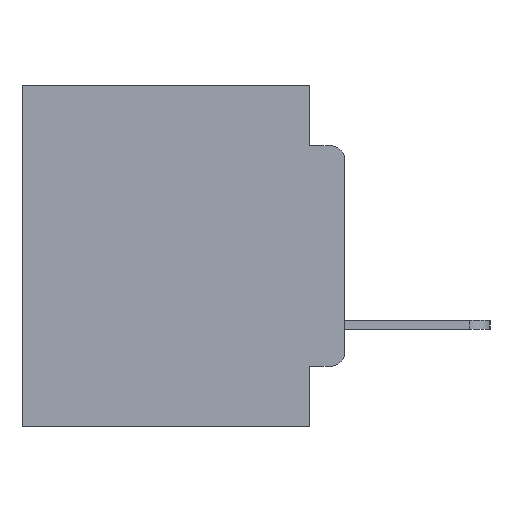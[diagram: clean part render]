
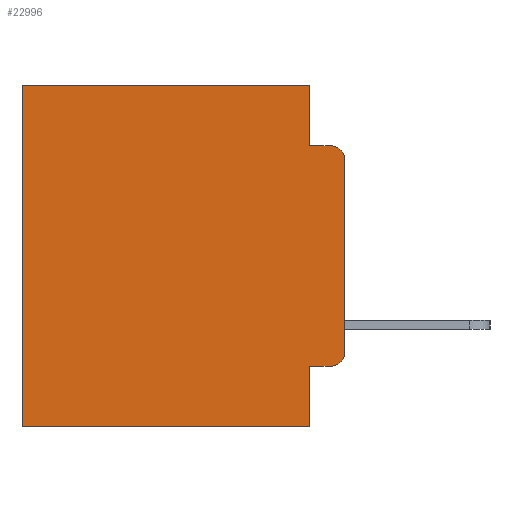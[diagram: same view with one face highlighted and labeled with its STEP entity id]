
A CAD part, left-side view. The second image highlights one B-rep face of the part: STEP entity #22996.
In plain terms, the highlighted planar face has unit normal (-1, 0, 0).
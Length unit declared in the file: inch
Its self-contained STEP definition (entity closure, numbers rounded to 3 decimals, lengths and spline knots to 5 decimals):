
#23 = VERTEX_POINT ( 'NONE', #1239 ) ;
#442 = CARTESIAN_POINT ( 'NONE',  ( 0.298, 0., 0. ) ) ;
#570 = ORIENTED_EDGE ( 'NONE', *, *, #21115, .T. ) ;
#1135 = DIRECTION ( 'NONE',  ( 0., -1., 0. ) ) ;
#1239 = CARTESIAN_POINT ( 'NONE',  ( 0.298, 0.051, -0.5 ) ) ;
#1432 = CARTESIAN_POINT ( 'NONE',  ( 0.298, 0.473, 0. ) ) ;
#1593 = CARTESIAN_POINT ( 'NONE',  ( 0.298, 0., 0. ) ) ;
#1882 = VERTEX_POINT ( 'NONE', #14518 ) ;
#2897 = CARTESIAN_POINT ( 'NONE',  ( 0.298, 0.051, -0.4115 ) ) ;
#2949 = VECTOR ( 'NONE', #7636, 39.37008 ) ;
#3294 = EDGE_CURVE ( 'NONE', #1882, #23, #17187, .T. ) ;
#3575 = VERTEX_POINT ( 'NONE', #11577 ) ;
#3702 = VECTOR ( 'NONE', #11290, 39.37008 ) ;
#5609 = VERTEX_POINT ( 'NONE', #14919 ) ;
#5889 = VERTEX_POINT ( 'NONE', #14248 ) ;
#6291 = CARTESIAN_POINT ( 'NONE',  ( 0.298, 0., -0.5 ) ) ;
#6502 = EDGE_CURVE ( 'NONE', #13504, #9636, #10635, .T. ) ;
#6533 = DIRECTION ( 'NONE',  ( 0., 0., -1. ) ) ;
#6785 = VECTOR ( 'NONE', #25525, 39.37008 ) ;
#6949 = LINE ( 'NONE', #1432, #23338 ) ;
#7346 = EDGE_LOOP ( 'NONE', ( #13256, #25888, #21569, #10869, #22143, #14944, #15572, #26911, #570, #9827 ) ) ;
#7636 = DIRECTION ( 'NONE',  ( 0., 1., 0. ) ) ;
#8042 = VERTEX_POINT ( 'NONE', #13746 ) ;
#9636 = VERTEX_POINT ( 'NONE', #17808 ) ;
#9827 = ORIENTED_EDGE ( 'NONE', *, *, #24387, .T. ) ;
#9970 = LINE ( 'NONE', #2897, #3702 ) ;
#10318 = DIRECTION ( 'NONE',  ( 0., 0., -1. ) ) ;
#10627 = CARTESIAN_POINT ( 'NONE',  ( 0.298, 0., -0.1085 ) ) ;
#10635 = LINE ( 'NONE', #24215, #12045 ) ;
#10776 = DIRECTION ( 'NONE',  ( 0., 0., -1. ) ) ;
#10869 = ORIENTED_EDGE ( 'NONE', *, *, #6502, .F. ) ;
#11014 = CIRCLE ( 'NONE', #19292, 0.02 ) ;
#11290 = DIRECTION ( 'NONE',  ( 0., -1., 0. ) ) ;
#11460 = VECTOR ( 'NONE', #1135, 39.37008 ) ;
#11577 = CARTESIAN_POINT ( 'NONE',  ( 0.298, 0.473, -0.5 ) ) ;
#11649 = VECTOR ( 'NONE', #23100, 39.37008 ) ;
#12045 = VECTOR ( 'NONE', #20986, 39.37008 ) ;
#12156 = LINE ( 'NONE', #15695, #11460 ) ;
#12810 = VECTOR ( 'NONE', #17911, 39.37008 ) ;
#13256 = ORIENTED_EDGE ( 'NONE', *, *, #20235, .F. ) ;
#13476 = LINE ( 'NONE', #442, #12810 ) ;
#13504 = VERTEX_POINT ( 'NONE', #20116 ) ;
#13746 = CARTESIAN_POINT ( 'NONE',  ( 0.298, 0.473, 0. ) ) ;
#14053 = VERTEX_POINT ( 'NONE', #10627 ) ;
#14248 = CARTESIAN_POINT ( 'NONE',  ( 0.298, 0.02, -0.0885 ) ) ;
#14318 = AXIS2_PLACEMENT_3D ( 'NONE', #15518, #20570, #21226 ) ;
#14518 = CARTESIAN_POINT ( 'NONE',  ( 0.298, 0.051, -0.4115 ) ) ;
#14919 = CARTESIAN_POINT ( 'NONE',  ( 0.298, 0., -0.3915 ) ) ;
#14944 = ORIENTED_EDGE ( 'NONE', *, *, #19282, .T. ) ;
#15074 = LINE ( 'NONE', #6291, #2949 ) ;
#15098 = CIRCLE ( 'NONE', #21481, 0.02 ) ;
#15518 = CARTESIAN_POINT ( 'NONE',  ( 0.298, 0., 0. ) ) ;
#15572 = ORIENTED_EDGE ( 'NONE', *, *, #25044, .F. ) ;
#15695 = CARTESIAN_POINT ( 'NONE',  ( 0.298, 0.051, -0.0885 ) ) ;
#17187 = LINE ( 'NONE', #21419, #11649 ) ;
#17793 = CARTESIAN_POINT ( 'NONE',  ( 0.298, 0.02, -0.4115 ) ) ;
#17808 = CARTESIAN_POINT ( 'NONE',  ( 0.298, 0.051, -0.0885 ) ) ;
#17911 = DIRECTION ( 'NONE',  ( 0., 0., -1. ) ) ;
#18573 = VERTEX_POINT ( 'NONE', #17793 ) ;
#18600 = DIRECTION ( 'NONE',  ( -1., 0., 0. ) ) ;
#18780 = CARTESIAN_POINT ( 'NONE',  ( 0.298, 0.02, -0.1085 ) ) ;
#19282 = EDGE_CURVE ( 'NONE', #8042, #3575, #6949, .T. ) ;
#19292 = AXIS2_PLACEMENT_3D ( 'NONE', #18780, #18600, #6533 ) ;
#19779 = EDGE_CURVE ( 'NONE', #9636, #5889, #12156, .T. ) ;
#20055 = PLANE ( 'NONE',  #14318 ) ;
#20061 = CARTESIAN_POINT ( 'NONE',  ( 0.298, 0.02, -0.3915 ) ) ;
#20116 = CARTESIAN_POINT ( 'NONE',  ( 0.298, 0.051, 0. ) ) ;
#20235 = EDGE_CURVE ( 'NONE', #14053, #5609, #13476, .T. ) ;
#20570 = DIRECTION ( 'NONE',  ( 1., 0., 0. ) ) ;
#20986 = DIRECTION ( 'NONE',  ( 0., 0., -1. ) ) ;
#21115 = EDGE_CURVE ( 'NONE', #1882, #18573, #9970, .T. ) ;
#21226 = DIRECTION ( 'NONE',  ( 0., 0., -1. ) ) ;
#21419 = CARTESIAN_POINT ( 'NONE',  ( 0.298, 0.051, 0. ) ) ;
#21481 = AXIS2_PLACEMENT_3D ( 'NONE', #20061, #25992, #10318 ) ;
#21569 = ORIENTED_EDGE ( 'NONE', *, *, #19779, .F. ) ;
#22143 = ORIENTED_EDGE ( 'NONE', *, *, #25555, .T. ) ;
#22996 = ADVANCED_FACE ( 'NONE', ( #26152 ), #20055, .F. ) ;
#23100 = DIRECTION ( 'NONE',  ( 0., 0., -1. ) ) ;
#23338 = VECTOR ( 'NONE', #10776, 39.37008 ) ;
#24215 = CARTESIAN_POINT ( 'NONE',  ( 0.298, 0.051, 0. ) ) ;
#24387 = EDGE_CURVE ( 'NONE', #18573, #5609, #15098, .T. ) ;
#25044 = EDGE_CURVE ( 'NONE', #23, #3575, #15074, .T. ) ;
#25275 = EDGE_CURVE ( 'NONE', #14053, #5889, #11014, .T. ) ;
#25525 = DIRECTION ( 'NONE',  ( 0., 1., 0. ) ) ;
#25555 = EDGE_CURVE ( 'NONE', #13504, #8042, #26755, .T. ) ;
#25888 = ORIENTED_EDGE ( 'NONE', *, *, #25275, .T. ) ;
#25992 = DIRECTION ( 'NONE',  ( -1., 0., 0. ) ) ;
#26152 = FACE_OUTER_BOUND ( 'NONE', #7346, .T. ) ;
#26755 = LINE ( 'NONE', #1593, #6785 ) ;
#26911 = ORIENTED_EDGE ( 'NONE', *, *, #3294, .F. ) ;
